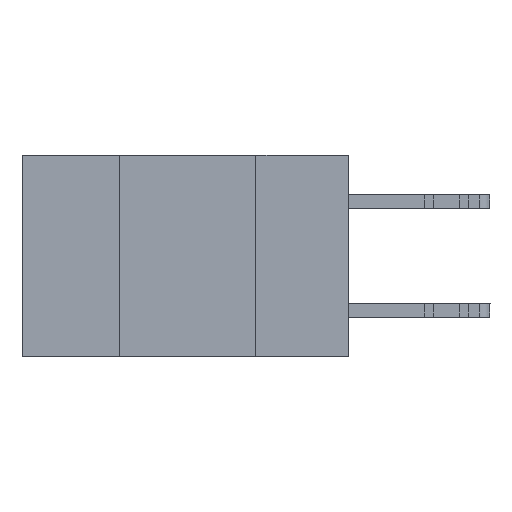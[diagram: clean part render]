
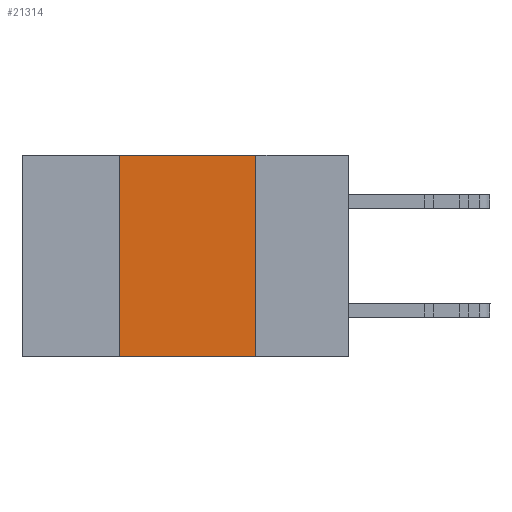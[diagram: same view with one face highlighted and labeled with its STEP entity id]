
A CAD part, left-side view. The second image highlights one B-rep face of the part: STEP entity #21314.
In plain terms, the highlighted planar face has unit normal (-1, 0, 0).
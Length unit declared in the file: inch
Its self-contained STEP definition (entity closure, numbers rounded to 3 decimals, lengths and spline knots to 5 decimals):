
#360 = EDGE_CURVE ( 'NONE', #17282, #13712, #24932, .T. ) ;
#500 = VERTEX_POINT ( 'NONE', #14538 ) ;
#1571 = DIRECTION ( 'NONE',  ( 0., 0., -1. ) ) ;
#1870 = CARTESIAN_POINT ( 'NONE',  ( 0., 0.6, -0.37 ) ) ;
#2706 = LINE ( 'NONE', #12899, #20585 ) ;
#2744 = CARTESIAN_POINT ( 'NONE',  ( 0., 0.17, -0.37 ) ) ;
#4341 = AXIS2_PLACEMENT_3D ( 'NONE', #6320, #22659, #8650 ) ;
#5543 = ORIENTED_EDGE ( 'NONE', *, *, #26298, .F. ) ;
#6320 = CARTESIAN_POINT ( 'NONE',  ( 0., 0.6, 0. ) ) ;
#7624 = EDGE_CURVE ( 'NONE', #8273, #500, #2706, .T. ) ;
#7665 = CARTESIAN_POINT ( 'NONE',  ( 0., 0.42, -0.37 ) ) ;
#8273 = VERTEX_POINT ( 'NONE', #19789 ) ;
#8650 = DIRECTION ( 'NONE',  ( 0., 0., -1. ) ) ;
#9827 = ORIENTED_EDGE ( 'NONE', *, *, #18110, .F. ) ;
#10396 = VECTOR ( 'NONE', #22066, 39.37008 ) ;
#11688 = ORIENTED_EDGE ( 'NONE', *, *, #7624, .F. ) ;
#12899 = CARTESIAN_POINT ( 'NONE',  ( 0., 0.6, 0. ) ) ;
#13494 = FACE_OUTER_BOUND ( 'NONE', #25591, .T. ) ;
#13712 = VERTEX_POINT ( 'NONE', #2744 ) ;
#14538 = CARTESIAN_POINT ( 'NONE',  ( 0., 0.17, 0. ) ) ;
#15217 = DIRECTION ( 'NONE',  ( 0., -1., 0. ) ) ;
#15309 = DIRECTION ( 'NONE',  ( 0., -1., 0. ) ) ;
#16364 = LINE ( 'NONE', #27110, #22570 ) ;
#16386 = ORIENTED_EDGE ( 'NONE', *, *, #360, .T. ) ;
#17282 = VERTEX_POINT ( 'NONE', #7665 ) ;
#18110 = EDGE_CURVE ( 'NONE', #17282, #8273, #28920, .T. ) ;
#19732 = CARTESIAN_POINT ( 'NONE',  ( 0., 0.42, 0. ) ) ;
#19789 = CARTESIAN_POINT ( 'NONE',  ( 0., 0.42, 0. ) ) ;
#20346 = PLANE ( 'NONE',  #4341 ) ;
#20585 = VECTOR ( 'NONE', #15217, 39.37008 ) ;
#21314 = ADVANCED_FACE ( 'NONE', ( #13494 ), #20346, .F. ) ;
#22066 = DIRECTION ( 'NONE',  ( 0., 0., 1. ) ) ;
#22570 = VECTOR ( 'NONE', #1571, 39.37008 ) ;
#22659 = DIRECTION ( 'NONE',  ( 1., 0., 0. ) ) ;
#24217 = VECTOR ( 'NONE', #15309, 39.37008 ) ;
#24932 = LINE ( 'NONE', #1870, #24217 ) ;
#25591 = EDGE_LOOP ( 'NONE', ( #5543, #11688, #9827, #16386 ) ) ;
#26298 = EDGE_CURVE ( 'NONE', #500, #13712, #16364, .T. ) ;
#27110 = CARTESIAN_POINT ( 'NONE',  ( 0., 0.17, 0. ) ) ;
#28920 = LINE ( 'NONE', #19732, #10396 ) ;
